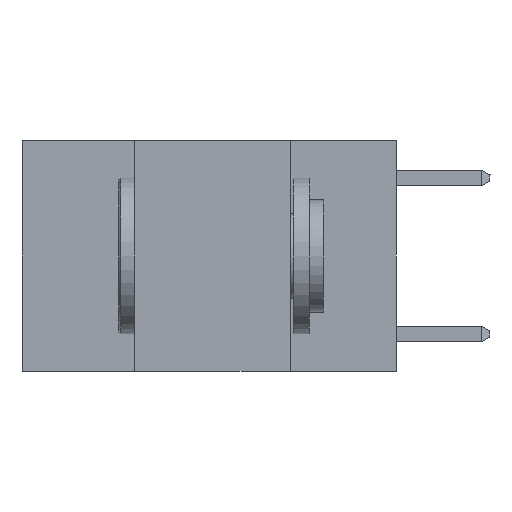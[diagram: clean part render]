
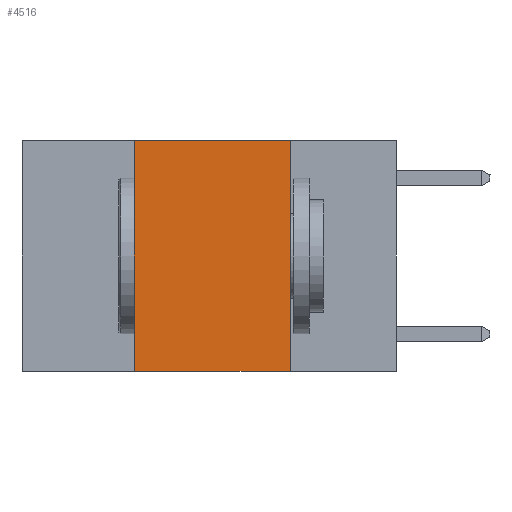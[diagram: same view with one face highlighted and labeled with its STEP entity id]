
A CAD part, left-side view. The second image highlights one B-rep face of the part: STEP entity #4516.
In plain terms, the highlighted planar face has unit normal (-1, 0, 0).
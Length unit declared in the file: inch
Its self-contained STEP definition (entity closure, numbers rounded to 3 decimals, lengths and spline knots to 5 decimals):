
#442 = LINE ( 'NONE', #1535, #4109 ) ;
#637 = CARTESIAN_POINT ( 'NONE',  ( 0., 0.6, -0.37 ) ) ;
#1333 = CARTESIAN_POINT ( 'NONE',  ( 0., 0.42, 0. ) ) ;
#1535 = CARTESIAN_POINT ( 'NONE',  ( 0., 0.6, 0. ) ) ;
#1538 = DIRECTION ( 'NONE',  ( 1., 0., 0. ) ) ;
#1998 = VECTOR ( 'NONE', #6578, 39.37008 ) ;
#2768 = EDGE_LOOP ( 'NONE', ( #7704, #3435, #7404, #6912 ) ) ;
#2819 = VECTOR ( 'NONE', #5982, 39.37008 ) ;
#3333 = FACE_OUTER_BOUND ( 'NONE', #2768, .T. ) ;
#3435 = ORIENTED_EDGE ( 'NONE', *, *, #7689, .F. ) ;
#3826 = CARTESIAN_POINT ( 'NONE',  ( 0., 0.6, 0. ) ) ;
#3952 = CARTESIAN_POINT ( 'NONE',  ( 0., 0.17, -0.37 ) ) ;
#4109 = VECTOR ( 'NONE', #7457, 39.37008 ) ;
#4400 = DIRECTION ( 'NONE',  ( 0., 0., -1. ) ) ;
#4516 = ADVANCED_FACE ( 'NONE', ( #3333 ), #9448, .F. ) ;
#4634 = VERTEX_POINT ( 'NONE', #9009 ) ;
#4983 = AXIS2_PLACEMENT_3D ( 'NONE', #3826, #1538, #6761 ) ;
#5944 = EDGE_CURVE ( 'NONE', #6374, #7858, #7067, .T. ) ;
#5982 = DIRECTION ( 'NONE',  ( 0., -1., 0. ) ) ;
#6374 = VERTEX_POINT ( 'NONE', #8925 ) ;
#6578 = DIRECTION ( 'NONE',  ( 0., 0., 1. ) ) ;
#6761 = DIRECTION ( 'NONE',  ( 0., 0., -1. ) ) ;
#6843 = EDGE_CURVE ( 'NONE', #4634, #7490, #9398, .T. ) ;
#6912 = ORIENTED_EDGE ( 'NONE', *, *, #7635, .T. ) ;
#7067 = LINE ( 'NONE', #7949, #8649 ) ;
#7404 = ORIENTED_EDGE ( 'NONE', *, *, #6843, .F. ) ;
#7457 = DIRECTION ( 'NONE',  ( 0., -1., 0. ) ) ;
#7490 = VERTEX_POINT ( 'NONE', #8580 ) ;
#7635 = EDGE_CURVE ( 'NONE', #4634, #7858, #8359, .T. ) ;
#7689 = EDGE_CURVE ( 'NONE', #7490, #6374, #442, .T. ) ;
#7704 = ORIENTED_EDGE ( 'NONE', *, *, #5944, .F. ) ;
#7858 = VERTEX_POINT ( 'NONE', #3952 ) ;
#7949 = CARTESIAN_POINT ( 'NONE',  ( 0., 0.17, 0. ) ) ;
#8359 = LINE ( 'NONE', #637, #2819 ) ;
#8580 = CARTESIAN_POINT ( 'NONE',  ( 0., 0.42, 0. ) ) ;
#8649 = VECTOR ( 'NONE', #4400, 39.37008 ) ;
#8925 = CARTESIAN_POINT ( 'NONE',  ( 0., 0.17, 0. ) ) ;
#9009 = CARTESIAN_POINT ( 'NONE',  ( 0., 0.42, -0.37 ) ) ;
#9398 = LINE ( 'NONE', #1333, #1998 ) ;
#9448 = PLANE ( 'NONE',  #4983 ) ;
